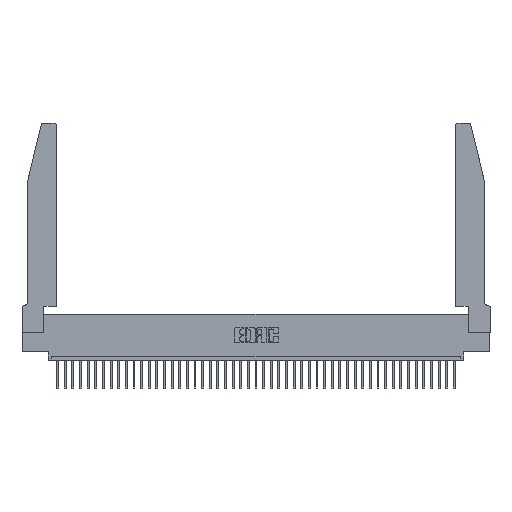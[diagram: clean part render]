
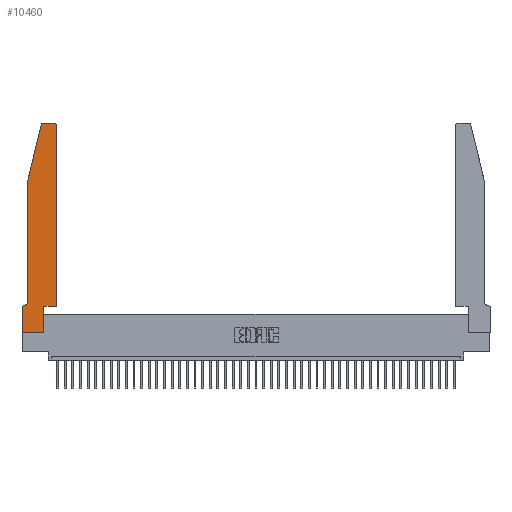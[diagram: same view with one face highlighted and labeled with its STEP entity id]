
A CAD part, top view. The second image highlights one B-rep face of the part: STEP entity #10460.
In plain terms, the highlighted planar face has unit normal (0, 0, 1).
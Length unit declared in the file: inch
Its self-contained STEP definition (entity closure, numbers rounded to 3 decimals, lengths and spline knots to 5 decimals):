
#1036 = DIRECTION ( 'NONE',  ( -1., 0., 0. ) ) ;
#1647 = CARTESIAN_POINT ( 'NONE',  ( 0., 0.35, 0.37 ) ) ;
#1934 = VECTOR ( 'NONE', #14905, 39.37008 ) ;
#3461 = EDGE_CURVE ( 'NONE', #17553, #38057, #18532, .T. ) ;
#3677 = CARTESIAN_POINT ( 'NONE',  ( 0., 0., 0.37 ) ) ;
#5078 = CARTESIAN_POINT ( 'NONE',  ( 0.0755, 2., 0.37 ) ) ;
#6199 = VERTEX_POINT ( 'NONE', #41448 ) ;
#6362 = DIRECTION ( 'NONE',  ( 1., 0., 0. ) ) ;
#6420 = DIRECTION ( 'NONE',  ( 0., 1., 0. ) ) ;
#6637 = DIRECTION ( 'NONE',  ( 0., -1., 0. ) ) ;
#6693 = VECTOR ( 'NONE', #22109, 39.37008 ) ;
#6895 = FACE_OUTER_BOUND ( 'NONE', #8968, .T. ) ;
#7207 = CARTESIAN_POINT ( 'NONE',  ( 0.2605, 2.75, 0.37 ) ) ;
#7665 = VERTEX_POINT ( 'NONE', #26191 ) ;
#8166 = CARTESIAN_POINT ( 'NONE',  ( 0.0755, 0.42, 0.37 ) ) ;
#8433 = EDGE_CURVE ( 'NONE', #7665, #42372, #38424, .T. ) ;
#8520 = ORIENTED_EDGE ( 'NONE', *, *, #8433, .T. ) ;
#8713 = CARTESIAN_POINT ( 'NONE',  ( 0.4505, 0.35, 0.37 ) ) ;
#8968 = EDGE_LOOP ( 'NONE', ( #8520, #13847, #13163, #18065, #23134, #13943, #33314, #18346, #43233, #19924, #24031, #29917 ) ) ;
#10255 = CARTESIAN_POINT ( 'NONE',  ( 0.284, 2.72, 0.37 ) ) ;
#10460 = ADVANCED_FACE ( 'NONE', ( #6895 ), #40457, .T. ) ;
#10676 = VECTOR ( 'NONE', #6637, 39.37008 ) ;
#11212 = CARTESIAN_POINT ( 'NONE',  ( 0.4505, 0.35, 0.37 ) ) ;
#11384 = LINE ( 'NONE', #8713, #6693 ) ;
#11428 = LINE ( 'NONE', #11212, #27635 ) ;
#11466 = DIRECTION ( 'NONE',  ( 1., 0., 0. ) ) ;
#12029 = VERTEX_POINT ( 'NONE', #1647 ) ;
#12820 = CARTESIAN_POINT ( 'NONE',  ( 0.25487, 2.72718, 0.37 ) ) ;
#13121 = EDGE_CURVE ( 'NONE', #42372, #17553, #40885, .T. ) ;
#13133 = CARTESIAN_POINT ( 'NONE',  ( 0.2865, 0.35, 0.37 ) ) ;
#13163 = ORIENTED_EDGE ( 'NONE', *, *, #3461, .T. ) ;
#13353 = LINE ( 'NONE', #13133, #32670 ) ;
#13656 = CARTESIAN_POINT ( 'NONE',  ( 0., 0., 0.37 ) ) ;
#13847 = ORIENTED_EDGE ( 'NONE', *, *, #13121, .T. ) ;
#13887 = DIRECTION ( 'NONE',  ( 0., 0., 1. ) ) ;
#13943 = ORIENTED_EDGE ( 'NONE', *, *, #25526, .T. ) ;
#14905 = DIRECTION ( 'NONE',  ( 0., -1., 0. ) ) ;
#15319 = AXIS2_PLACEMENT_3D ( 'NONE', #34522, #40996, #11466 ) ;
#15666 = VERTEX_POINT ( 'NONE', #42055 ) ;
#16020 = EDGE_CURVE ( 'NONE', #6199, #43010, #11428, .T. ) ;
#17268 = DIRECTION ( 'NONE',  ( 0., 0., -1. ) ) ;
#17455 = CIRCLE ( 'NONE', #15319, 0.03 ) ;
#17553 = VERTEX_POINT ( 'NONE', #12820 ) ;
#17557 = VECTOR ( 'NONE', #1036, 39.37008 ) ;
#18065 = ORIENTED_EDGE ( 'NONE', *, *, #40524, .T. ) ;
#18346 = ORIENTED_EDGE ( 'NONE', *, *, #24892, .T. ) ;
#18532 = LINE ( 'NONE', #5078, #23195 ) ;
#19527 = LINE ( 'NONE', #3677, #10676 ) ;
#19549 = VERTEX_POINT ( 'NONE', #20207 ) ;
#19924 = ORIENTED_EDGE ( 'NONE', *, *, #16020, .T. ) ;
#20207 = CARTESIAN_POINT ( 'NONE',  ( 0.0055, 0.35, 0.37 ) ) ;
#20315 = LINE ( 'NONE', #29561, #28180 ) ;
#20747 = CARTESIAN_POINT ( 'NONE',  ( 0.0755, 2., 0.37 ) ) ;
#21362 = EDGE_CURVE ( 'NONE', #34096, #19549, #36714, .T. ) ;
#21416 = CARTESIAN_POINT ( 'NONE',  ( 0.0755, 2., 0.37 ) ) ;
#21686 = VERTEX_POINT ( 'NONE', #42632 ) ;
#22042 = DIRECTION ( 'NONE',  ( -1., 0., 0. ) ) ;
#22109 = DIRECTION ( 'NONE',  ( 0., 1., 0. ) ) ;
#23134 = ORIENTED_EDGE ( 'NONE', *, *, #21362, .T. ) ;
#23195 = VECTOR ( 'NONE', #28586, 39.37008 ) ;
#23639 = AXIS2_PLACEMENT_3D ( 'NONE', #23675, #17268, #27057 ) ;
#23675 = CARTESIAN_POINT ( 'NONE',  ( 0.0055, 0.42, 0.37 ) ) ;
#24031 = ORIENTED_EDGE ( 'NONE', *, *, #35952, .T. ) ;
#24892 = EDGE_CURVE ( 'NONE', #26869, #21686, #20315, .T. ) ;
#25526 = EDGE_CURVE ( 'NONE', #19549, #12029, #38022, .T. ) ;
#26191 = CARTESIAN_POINT ( 'NONE',  ( 0.4205, 2.75, 0.37 ) ) ;
#26869 = VERTEX_POINT ( 'NONE', #13656 ) ;
#27057 = DIRECTION ( 'NONE',  ( -1., 0., 0. ) ) ;
#27300 = DIRECTION ( 'NONE',  ( 1., 0., 0. ) ) ;
#27635 = VECTOR ( 'NONE', #34259, 39.37008 ) ;
#28180 = VECTOR ( 'NONE', #6362, 39.37008 ) ;
#28586 = DIRECTION ( 'NONE',  ( -0.239, -0.971, 0. ) ) ;
#29561 = CARTESIAN_POINT ( 'NONE',  ( 0., 0., 0.37 ) ) ;
#29917 = ORIENTED_EDGE ( 'NONE', *, *, #32157, .T. ) ;
#30521 = CARTESIAN_POINT ( 'NONE',  ( 0., 0.35, 0.37 ) ) ;
#31256 = EDGE_CURVE ( 'NONE', #21686, #6199, #13353, .T. ) ;
#32157 = EDGE_CURVE ( 'NONE', #15666, #7665, #17455, .T. ) ;
#32670 = VECTOR ( 'NONE', #6420, 39.37008 ) ;
#33314 = ORIENTED_EDGE ( 'NONE', *, *, #42064, .T. ) ;
#34096 = VERTEX_POINT ( 'NONE', #8166 ) ;
#34259 = DIRECTION ( 'NONE',  ( 1., 0., 0. ) ) ;
#34522 = CARTESIAN_POINT ( 'NONE',  ( 0.4205, 2.72, 0.37 ) ) ;
#34796 = AXIS2_PLACEMENT_3D ( 'NONE', #30521, #13887, #27300 ) ;
#35952 = EDGE_CURVE ( 'NONE', #43010, #15666, #11384, .T. ) ;
#36388 = LINE ( 'NONE', #21416, #1934 ) ;
#36714 = CIRCLE ( 'NONE', #23639, 0.07 ) ;
#38022 = LINE ( 'NONE', #42097, #42221 ) ;
#38057 = VERTEX_POINT ( 'NONE', #20747 ) ;
#38424 = LINE ( 'NONE', #7207, #17557 ) ;
#39265 = CARTESIAN_POINT ( 'NONE',  ( 0.284, 2.75, 0.37 ) ) ;
#40162 = DIRECTION ( 'NONE',  ( 1., 0., 0. ) ) ;
#40457 = PLANE ( 'NONE',  #34796 ) ;
#40524 = EDGE_CURVE ( 'NONE', #38057, #34096, #36388, .T. ) ;
#40766 = DIRECTION ( 'NONE',  ( 0., 0., 1. ) ) ;
#40885 = CIRCLE ( 'NONE', #42395, 0.03 ) ;
#40996 = DIRECTION ( 'NONE',  ( 0., 0., 1. ) ) ;
#41448 = CARTESIAN_POINT ( 'NONE',  ( 0.2865, 0.35, 0.37 ) ) ;
#41456 = CARTESIAN_POINT ( 'NONE',  ( 0.4505, 0.35, 0.37 ) ) ;
#42055 = CARTESIAN_POINT ( 'NONE',  ( 0.4505, 2.72, 0.37 ) ) ;
#42064 = EDGE_CURVE ( 'NONE', #12029, #26869, #19527, .T. ) ;
#42097 = CARTESIAN_POINT ( 'NONE',  ( 0.0755, 0.35, 0.37 ) ) ;
#42221 = VECTOR ( 'NONE', #22042, 39.37008 ) ;
#42372 = VERTEX_POINT ( 'NONE', #39265 ) ;
#42395 = AXIS2_PLACEMENT_3D ( 'NONE', #10255, #40766, #40162 ) ;
#42632 = CARTESIAN_POINT ( 'NONE',  ( 0.2865, 0., 0.37 ) ) ;
#43010 = VERTEX_POINT ( 'NONE', #41456 ) ;
#43233 = ORIENTED_EDGE ( 'NONE', *, *, #31256, .T. ) ;
